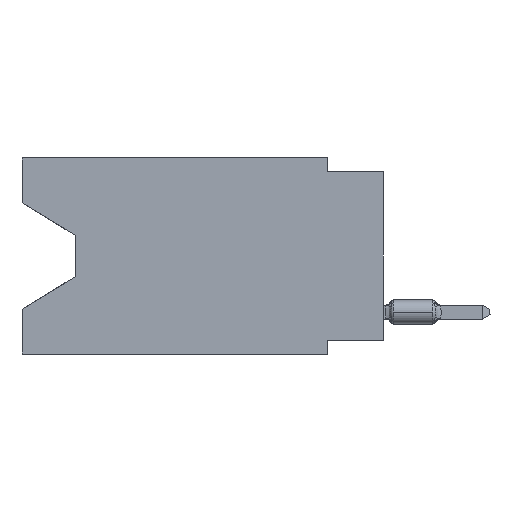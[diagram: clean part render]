
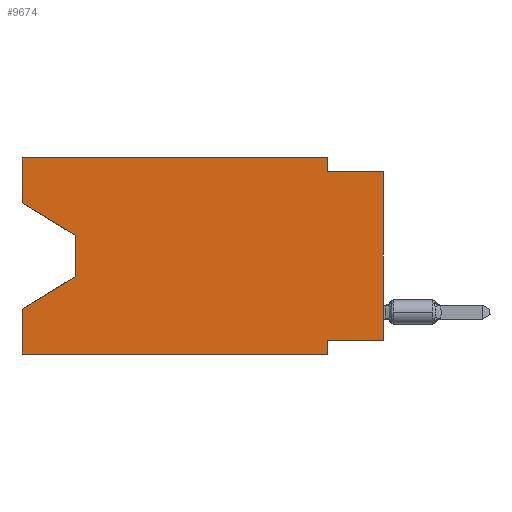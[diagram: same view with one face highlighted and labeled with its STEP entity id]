
A CAD part, left-side view. The second image highlights one B-rep face of the part: STEP entity #9674.
In plain terms, the highlighted planar face has unit normal (-1, 0, 0).
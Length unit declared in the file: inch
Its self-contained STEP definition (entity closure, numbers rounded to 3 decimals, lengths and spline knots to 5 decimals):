
#109 = CARTESIAN_POINT ( 'NONE',  ( 0., 0.1, 0. ) ) ;
#460 = VERTEX_POINT ( 'NONE', #11275 ) ;
#568 = EDGE_CURVE ( 'NONE', #11753, #30225, #23878, .T. ) ;
#2260 = VERTEX_POINT ( 'NONE', #33941 ) ;
#2361 = ORIENTED_EDGE ( 'NONE', *, *, #7292, .T. ) ;
#2637 = VECTOR ( 'NONE', #9763, 39.37008 ) ;
#2750 = VECTOR ( 'NONE', #29401, 39.37008 ) ;
#2970 = ORIENTED_EDGE ( 'NONE', *, *, #29783, .T. ) ;
#3086 = DIRECTION ( 'NONE',  ( 0., 0., -1. ) ) ;
#3186 = CARTESIAN_POINT ( 'NONE',  ( 0., 0.645, -0.08025 ) ) ;
#3513 = LINE ( 'NONE', #14006, #15220 ) ;
#3601 = ORIENTED_EDGE ( 'NONE', *, *, #568, .F. ) ;
#3693 = DIRECTION ( 'NONE',  ( 0., -0.855, -0.519 ) ) ;
#3783 = DIRECTION ( 'NONE',  ( 0., 0.855, -0.519 ) ) ;
#3833 = CARTESIAN_POINT ( 'NONE',  ( 0., 0.55, -0.138 ) ) ;
#4101 = VERTEX_POINT ( 'NONE', #7832 ) ;
#4423 = EDGE_LOOP ( 'NONE', ( #9745, #33421, #2361, #5327, #2970, #8048, #29178, #27126, #3601, #33999, #26572, #20825 ) ) ;
#5183 = EDGE_CURVE ( 'NONE', #20161, #30225, #8936, .T. ) ;
#5327 = ORIENTED_EDGE ( 'NONE', *, *, #28790, .F. ) ;
#5420 = VERTEX_POINT ( 'NONE', #3186 ) ;
#5550 = DIRECTION ( 'NONE',  ( 0., -1., 0. ) ) ;
#6286 = CARTESIAN_POINT ( 'NONE',  ( 0., 0.645, 0. ) ) ;
#6691 = VERTEX_POINT ( 'NONE', #3833 ) ;
#7292 = EDGE_CURVE ( 'NONE', #27737, #33184, #28306, .T. ) ;
#7832 = CARTESIAN_POINT ( 'NONE',  ( 0., 0.1, -0.325 ) ) ;
#7863 = VERTEX_POINT ( 'NONE', #109 ) ;
#8048 = ORIENTED_EDGE ( 'NONE', *, *, #31875, .F. ) ;
#8421 = DIRECTION ( 'NONE',  ( 1., 0., 0. ) ) ;
#8936 = LINE ( 'NONE', #19791, #27342 ) ;
#9674 = ADVANCED_FACE ( 'NONE', ( #13744 ), #16051, .F. ) ;
#9723 = DIRECTION ( 'NONE',  ( 0., 0., 1. ) ) ;
#9745 = ORIENTED_EDGE ( 'NONE', *, *, #31742, .T. ) ;
#9763 = DIRECTION ( 'NONE',  ( 0., 0., 1. ) ) ;
#10329 = CARTESIAN_POINT ( 'NONE',  ( 0., 0.645, -0.35 ) ) ;
#11275 = CARTESIAN_POINT ( 'NONE',  ( 0., 0.645, 0. ) ) ;
#11563 = VECTOR ( 'NONE', #30800, 39.37008 ) ;
#11753 = VERTEX_POINT ( 'NONE', #15405 ) ;
#11822 = VECTOR ( 'NONE', #25098, 39.37008 ) ;
#12343 = AXIS2_PLACEMENT_3D ( 'NONE', #24597, #8421, #3086 ) ;
#12571 = EDGE_CURVE ( 'NONE', #5420, #460, #23448, .T. ) ;
#12925 = CARTESIAN_POINT ( 'NONE',  ( 0., 0.1, -0.35 ) ) ;
#13005 = LINE ( 'NONE', #10329, #20224 ) ;
#13561 = CARTESIAN_POINT ( 'NONE',  ( 0., 0., -0.325 ) ) ;
#13744 = FACE_OUTER_BOUND ( 'NONE', #4423, .T. ) ;
#13896 = LINE ( 'NONE', #13561, #11822 ) ;
#14006 = CARTESIAN_POINT ( 'NONE',  ( 0., 0.645, -0.08025 ) ) ;
#15220 = VECTOR ( 'NONE', #3693, 39.37008 ) ;
#15405 = CARTESIAN_POINT ( 'NONE',  ( 0., 0.1, -0.025 ) ) ;
#16051 = PLANE ( 'NONE',  #12343 ) ;
#17410 = CARTESIAN_POINT ( 'NONE',  ( 0., 0.55, -0.138 ) ) ;
#17591 = LINE ( 'NONE', #17410, #21989 ) ;
#18078 = CARTESIAN_POINT ( 'NONE',  ( 0., 0.645, 0. ) ) ;
#18206 = LINE ( 'NONE', #29204, #2750 ) ;
#18401 = VECTOR ( 'NONE', #26117, 39.37008 ) ;
#18733 = VECTOR ( 'NONE', #5550, 39.37008 ) ;
#18825 = CARTESIAN_POINT ( 'NONE',  ( 0., 0., -0.025 ) ) ;
#19209 = VECTOR ( 'NONE', #3783, 39.37008 ) ;
#19791 = CARTESIAN_POINT ( 'NONE',  ( 0., 0., 0. ) ) ;
#19976 = LINE ( 'NONE', #6286, #11563 ) ;
#20116 = CARTESIAN_POINT ( 'NONE',  ( 0., 0.55, -0.212 ) ) ;
#20161 = VERTEX_POINT ( 'NONE', #23290 ) ;
#20224 = VECTOR ( 'NONE', #24015, 39.37008 ) ;
#20825 = ORIENTED_EDGE ( 'NONE', *, *, #12571, .F. ) ;
#21722 = CARTESIAN_POINT ( 'NONE',  ( 0., 0., -0.025 ) ) ;
#21989 = VECTOR ( 'NONE', #33758, 39.37008 ) ;
#23290 = CARTESIAN_POINT ( 'NONE',  ( 0., 0., -0.325 ) ) ;
#23448 = LINE ( 'NONE', #34115, #2637 ) ;
#23878 = LINE ( 'NONE', #21722, #18733 ) ;
#24015 = DIRECTION ( 'NONE',  ( 0., -1., 0. ) ) ;
#24597 = CARTESIAN_POINT ( 'NONE',  ( 0., 0.645, 0. ) ) ;
#25098 = DIRECTION ( 'NONE',  ( 0., 1., 0. ) ) ;
#25379 = EDGE_CURVE ( 'NONE', #20161, #4101, #13896, .T. ) ;
#26117 = DIRECTION ( 'NONE',  ( 0., 0., -1. ) ) ;
#26273 = LINE ( 'NONE', #26635, #18401 ) ;
#26572 = ORIENTED_EDGE ( 'NONE', *, *, #34958, .F. ) ;
#26635 = CARTESIAN_POINT ( 'NONE',  ( 0., 0.1, 0. ) ) ;
#27126 = ORIENTED_EDGE ( 'NONE', *, *, #5183, .T. ) ;
#27342 = VECTOR ( 'NONE', #30629, 39.37008 ) ;
#27520 = EDGE_CURVE ( 'NONE', #7863, #11753, #26273, .T. ) ;
#27737 = VERTEX_POINT ( 'NONE', #20116 ) ;
#28306 = LINE ( 'NONE', #34804, #19209 ) ;
#28653 = VECTOR ( 'NONE', #9723, 39.37008 ) ;
#28790 = EDGE_CURVE ( 'NONE', #2260, #33184, #34078, .T. ) ;
#29178 = ORIENTED_EDGE ( 'NONE', *, *, #25379, .F. ) ;
#29204 = CARTESIAN_POINT ( 'NONE',  ( 0., 0.1, -0.35 ) ) ;
#29401 = DIRECTION ( 'NONE',  ( 0., 0., -1. ) ) ;
#29783 = EDGE_CURVE ( 'NONE', #2260, #33060, #13005, .T. ) ;
#30225 = VERTEX_POINT ( 'NONE', #18825 ) ;
#30629 = DIRECTION ( 'NONE',  ( 0., 0., 1. ) ) ;
#30800 = DIRECTION ( 'NONE',  ( 0., -1., 0. ) ) ;
#31742 = EDGE_CURVE ( 'NONE', #5420, #6691, #3513, .T. ) ;
#31875 = EDGE_CURVE ( 'NONE', #4101, #33060, #18206, .T. ) ;
#32296 = CARTESIAN_POINT ( 'NONE',  ( 0., 0.645, -0.26975 ) ) ;
#32484 = EDGE_CURVE ( 'NONE', #6691, #27737, #17591, .T. ) ;
#33060 = VERTEX_POINT ( 'NONE', #12925 ) ;
#33184 = VERTEX_POINT ( 'NONE', #32296 ) ;
#33421 = ORIENTED_EDGE ( 'NONE', *, *, #32484, .T. ) ;
#33758 = DIRECTION ( 'NONE',  ( 0., 0., -1. ) ) ;
#33941 = CARTESIAN_POINT ( 'NONE',  ( 0., 0.645, -0.35 ) ) ;
#33999 = ORIENTED_EDGE ( 'NONE', *, *, #27520, .F. ) ;
#34078 = LINE ( 'NONE', #18078, #28653 ) ;
#34115 = CARTESIAN_POINT ( 'NONE',  ( 0., 0.645, 0. ) ) ;
#34804 = CARTESIAN_POINT ( 'NONE',  ( 0., 0.55, -0.212 ) ) ;
#34958 = EDGE_CURVE ( 'NONE', #460, #7863, #19976, .T. ) ;
